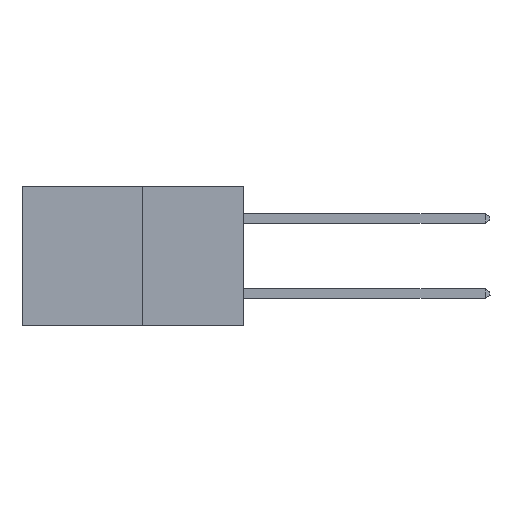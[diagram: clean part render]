
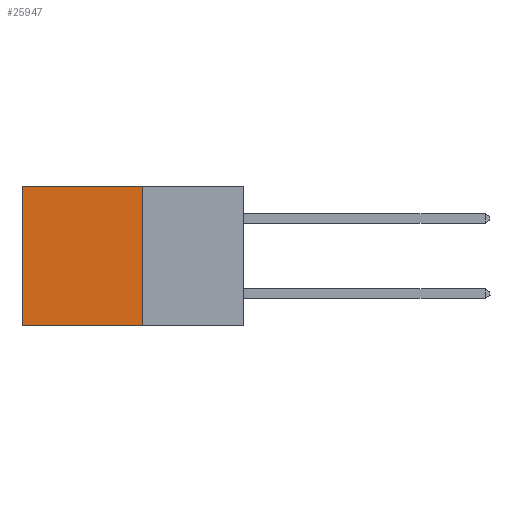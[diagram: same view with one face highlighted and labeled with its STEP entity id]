
A CAD part, left-side view. The second image highlights one B-rep face of the part: STEP entity #25947.
In plain terms, the highlighted planar face has unit normal (-1, 0, 0).
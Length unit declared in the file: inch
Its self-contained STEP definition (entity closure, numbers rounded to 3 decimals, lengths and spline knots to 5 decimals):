
#1150 = VECTOR ( 'NONE', #7032, 39.37008 ) ;
#1438 = EDGE_CURVE ( 'NONE', #5767, #32303, #34608, .T. ) ;
#2500 = EDGE_CURVE ( 'NONE', #23340, #17896, #16168, .T. ) ;
#3772 = PLANE ( 'NONE',  #35147 ) ;
#5767 = VERTEX_POINT ( 'NONE', #7856 ) ;
#6629 = CARTESIAN_POINT ( 'NONE',  ( 0.277, 0.27, -0.37 ) ) ;
#7032 = DIRECTION ( 'NONE',  ( 0., 1., 0. ) ) ;
#7528 = DIRECTION ( 'NONE',  ( 0., 0., -1. ) ) ;
#7856 = CARTESIAN_POINT ( 'NONE',  ( 0.277, 0.27, -0.37 ) ) ;
#9150 = CARTESIAN_POINT ( 'NONE',  ( 0.277, 0.59, 0. ) ) ;
#9494 = DIRECTION ( 'NONE',  ( 1., 0., 0. ) ) ;
#13279 = ORIENTED_EDGE ( 'NONE', *, *, #1438, .F. ) ;
#14259 = CARTESIAN_POINT ( 'NONE',  ( 0.277, 0.27, 0. ) ) ;
#16168 = LINE ( 'NONE', #14259, #1150 ) ;
#16229 = FACE_OUTER_BOUND ( 'NONE', #32275, .T. ) ;
#17394 = VECTOR ( 'NONE', #25250, 39.37008 ) ;
#17896 = VERTEX_POINT ( 'NONE', #9150 ) ;
#21412 = ORIENTED_EDGE ( 'NONE', *, *, #2500, .T. ) ;
#22238 = VECTOR ( 'NONE', #7528, 39.37008 ) ;
#23340 = VERTEX_POINT ( 'NONE', #35165 ) ;
#23389 = EDGE_CURVE ( 'NONE', #23340, #5767, #28788, .T. ) ;
#24321 = CARTESIAN_POINT ( 'NONE',  ( 0.277, 0.27, -0.37 ) ) ;
#24845 = LINE ( 'NONE', #33545, #17394 ) ;
#25250 = DIRECTION ( 'NONE',  ( 0., 0., -1. ) ) ;
#25947 = ADVANCED_FACE ( 'NONE', ( #16229 ), #3772, .F. ) ;
#27208 = VECTOR ( 'NONE', #27278, 39.37008 ) ;
#27278 = DIRECTION ( 'NONE',  ( 0., 1., 0. ) ) ;
#28580 = EDGE_CURVE ( 'NONE', #17896, #32303, #24845, .T. ) ;
#28788 = LINE ( 'NONE', #24321, #22238 ) ;
#29056 = DIRECTION ( 'NONE',  ( 0., 0., -1. ) ) ;
#31615 = ORIENTED_EDGE ( 'NONE', *, *, #28580, .T. ) ;
#32275 = EDGE_LOOP ( 'NONE', ( #31615, #13279, #33996, #21412 ) ) ;
#32303 = VERTEX_POINT ( 'NONE', #34087 ) ;
#33545 = CARTESIAN_POINT ( 'NONE',  ( 0.277, 0.59, -0.37 ) ) ;
#33996 = ORIENTED_EDGE ( 'NONE', *, *, #23389, .F. ) ;
#34087 = CARTESIAN_POINT ( 'NONE',  ( 0.277, 0.59, -0.37 ) ) ;
#34608 = LINE ( 'NONE', #35017, #27208 ) ;
#35017 = CARTESIAN_POINT ( 'NONE',  ( 0.277, 0.27, -0.37 ) ) ;
#35147 = AXIS2_PLACEMENT_3D ( 'NONE', #6629, #9494, #29056 ) ;
#35165 = CARTESIAN_POINT ( 'NONE',  ( 0.277, 0.27, 0. ) ) ;
